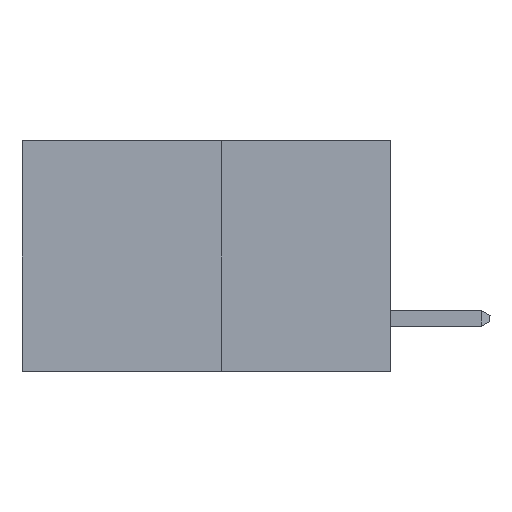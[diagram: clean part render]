
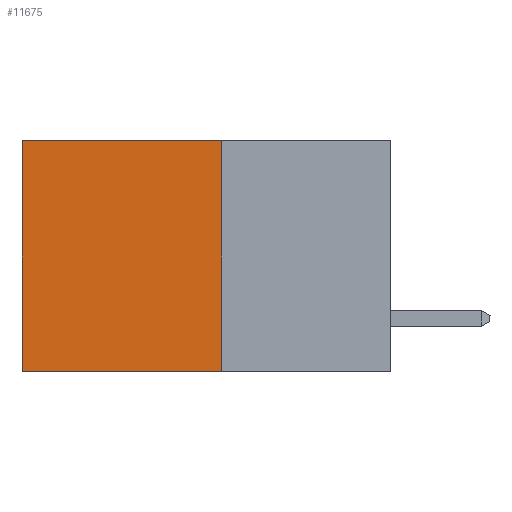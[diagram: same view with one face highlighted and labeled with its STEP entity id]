
A CAD part, left-side view. The second image highlights one B-rep face of the part: STEP entity #11675.
In plain terms, the highlighted planar face has unit normal (-1, 0, 0).
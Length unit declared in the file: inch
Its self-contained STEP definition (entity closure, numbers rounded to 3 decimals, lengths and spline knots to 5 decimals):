
#232 = CARTESIAN_POINT ( 'NONE',  ( 0.277, 0.59, -0.37 ) ) ;
#324 = ORIENTED_EDGE ( 'NONE', *, *, #8438, .F. ) ;
#609 = EDGE_CURVE ( 'NONE', #9566, #2872, #9296, .T. ) ;
#783 = EDGE_LOOP ( 'NONE', ( #810, #324, #836, #4742 ) ) ;
#810 = ORIENTED_EDGE ( 'NONE', *, *, #5627, .T. ) ;
#836 = ORIENTED_EDGE ( 'NONE', *, *, #609, .F. ) ;
#2601 = VERTEX_POINT ( 'NONE', #232 ) ;
#2604 = CARTESIAN_POINT ( 'NONE',  ( 0.277, 0.27, -0.37 ) ) ;
#2681 = CARTESIAN_POINT ( 'NONE',  ( 0.277, 0.27, -0.37 ) ) ;
#2872 = VERTEX_POINT ( 'NONE', #2604 ) ;
#3285 = EDGE_CURVE ( 'NONE', #9566, #6527, #10819, .T. ) ;
#3334 = VECTOR ( 'NONE', #5268, 39.37008 ) ;
#3800 = DIRECTION ( 'NONE',  ( 1., 0., 0. ) ) ;
#4716 = CARTESIAN_POINT ( 'NONE',  ( 0.277, 0.27, -0.37 ) ) ;
#4742 = ORIENTED_EDGE ( 'NONE', *, *, #3285, .T. ) ;
#5268 = DIRECTION ( 'NONE',  ( 0., 0., -1. ) ) ;
#5361 = CARTESIAN_POINT ( 'NONE',  ( 0.277, 0.27, 0. ) ) ;
#5441 = CARTESIAN_POINT ( 'NONE',  ( 0.277, 0.27, 0. ) ) ;
#5475 = DIRECTION ( 'NONE',  ( 0., 1., 0. ) ) ;
#5627 = EDGE_CURVE ( 'NONE', #6527, #2601, #9009, .T. ) ;
#6336 = CARTESIAN_POINT ( 'NONE',  ( 0.277, 0.59, -0.37 ) ) ;
#6361 = DIRECTION ( 'NONE',  ( 0., 0., -1. ) ) ;
#6509 = LINE ( 'NONE', #13032, #9066 ) ;
#6527 = VERTEX_POINT ( 'NONE', #11646 ) ;
#7608 = DIRECTION ( 'NONE',  ( 0., 1., 0. ) ) ;
#7662 = AXIS2_PLACEMENT_3D ( 'NONE', #2681, #3800, #11582 ) ;
#7897 = VECTOR ( 'NONE', #5475, 39.37008 ) ;
#8438 = EDGE_CURVE ( 'NONE', #2872, #2601, #6509, .T. ) ;
#9009 = LINE ( 'NONE', #6336, #10910 ) ;
#9066 = VECTOR ( 'NONE', #7608, 39.37008 ) ;
#9296 = LINE ( 'NONE', #4716, #3334 ) ;
#9378 = PLANE ( 'NONE',  #7662 ) ;
#9566 = VERTEX_POINT ( 'NONE', #5361 ) ;
#10819 = LINE ( 'NONE', #5441, #7897 ) ;
#10910 = VECTOR ( 'NONE', #6361, 39.37008 ) ;
#11582 = DIRECTION ( 'NONE',  ( 0., 0., -1. ) ) ;
#11646 = CARTESIAN_POINT ( 'NONE',  ( 0.277, 0.59, 0. ) ) ;
#11675 = ADVANCED_FACE ( 'NONE', ( #12281 ), #9378, .F. ) ;
#12281 = FACE_OUTER_BOUND ( 'NONE', #783, .T. ) ;
#13032 = CARTESIAN_POINT ( 'NONE',  ( 0.277, 0.27, -0.37 ) ) ;
